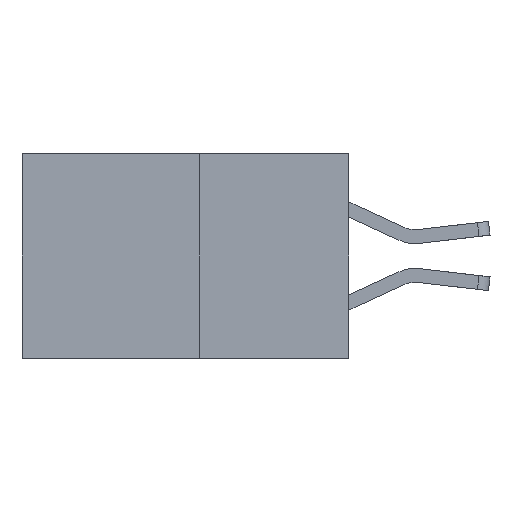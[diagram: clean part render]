
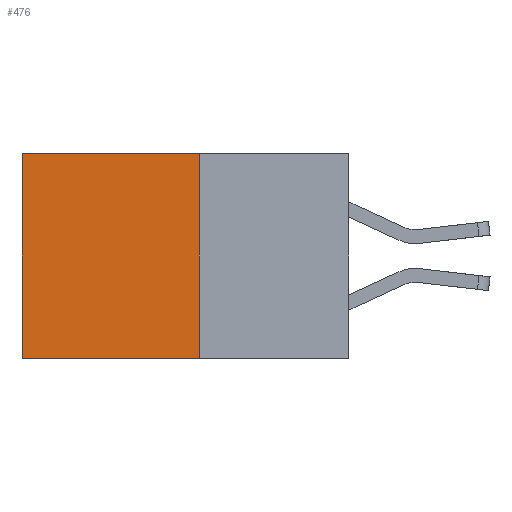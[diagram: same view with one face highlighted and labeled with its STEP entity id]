
A CAD part, left-side view. The second image highlights one B-rep face of the part: STEP entity #476.
In plain terms, the highlighted planar face has unit normal (-1, 0, 0).
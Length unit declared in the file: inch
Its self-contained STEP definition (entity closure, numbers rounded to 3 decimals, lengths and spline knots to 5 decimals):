
#105 = VERTEX_POINT ( 'NONE', #1297 ) ;
#317 = LINE ( 'NONE', #5984, #1931 ) ;
#476 = ADVANCED_FACE ( 'NONE', ( #6765 ), #1693, .F. ) ;
#794 = ORIENTED_EDGE ( 'NONE', *, *, #4523, .T. ) ;
#843 = ORIENTED_EDGE ( 'NONE', *, *, #1957, .F. ) ;
#1030 = DIRECTION ( 'NONE',  ( 0., 0., -1. ) ) ;
#1036 = DIRECTION ( 'NONE',  ( 0., 1., 0. ) ) ;
#1147 = ORIENTED_EDGE ( 'NONE', *, *, #6575, .F. ) ;
#1293 = DIRECTION ( 'NONE',  ( 0., 0., -1. ) ) ;
#1297 = CARTESIAN_POINT ( 'NONE',  ( 0.277, 0.27, -0.37 ) ) ;
#1533 = CARTESIAN_POINT ( 'NONE',  ( 0.277, 0.27, 0. ) ) ;
#1543 = ORIENTED_EDGE ( 'NONE', *, *, #7223, .T. ) ;
#1693 = PLANE ( 'NONE',  #6329 ) ;
#1805 = CARTESIAN_POINT ( 'NONE',  ( 0.277, 0.27, -0.37 ) ) ;
#1931 = VECTOR ( 'NONE', #6585, 39.37008 ) ;
#1957 = EDGE_CURVE ( 'NONE', #105, #7918, #4616, .T. ) ;
#3198 = VECTOR ( 'NONE', #4562, 39.37008 ) ;
#4405 = VECTOR ( 'NONE', #1036, 39.37008 ) ;
#4523 = EDGE_CURVE ( 'NONE', #5938, #7918, #7222, .T. ) ;
#4562 = DIRECTION ( 'NONE',  ( 0., 0., -1. ) ) ;
#4581 = CARTESIAN_POINT ( 'NONE',  ( 0.277, 0.59, -0.37 ) ) ;
#4616 = LINE ( 'NONE', #8134, #4405 ) ;
#4833 = CARTESIAN_POINT ( 'NONE',  ( 0.277, 0.27, -0.37 ) ) ;
#4920 = CARTESIAN_POINT ( 'NONE',  ( 0.277, 0.59, 0. ) ) ;
#5712 = VECTOR ( 'NONE', #1030, 39.37008 ) ;
#5874 = EDGE_LOOP ( 'NONE', ( #794, #843, #1147, #1543 ) ) ;
#5938 = VERTEX_POINT ( 'NONE', #4920 ) ;
#5984 = CARTESIAN_POINT ( 'NONE',  ( 0.277, 0.27, 0. ) ) ;
#6005 = CARTESIAN_POINT ( 'NONE',  ( 0.277, 0.59, -0.37 ) ) ;
#6329 = AXIS2_PLACEMENT_3D ( 'NONE', #1805, #7372, #1293 ) ;
#6368 = VERTEX_POINT ( 'NONE', #1533 ) ;
#6575 = EDGE_CURVE ( 'NONE', #6368, #105, #7285, .T. ) ;
#6585 = DIRECTION ( 'NONE',  ( 0., 1., 0. ) ) ;
#6765 = FACE_OUTER_BOUND ( 'NONE', #5874, .T. ) ;
#7222 = LINE ( 'NONE', #4581, #3198 ) ;
#7223 = EDGE_CURVE ( 'NONE', #6368, #5938, #317, .T. ) ;
#7285 = LINE ( 'NONE', #4833, #5712 ) ;
#7372 = DIRECTION ( 'NONE',  ( 1., 0., 0. ) ) ;
#7918 = VERTEX_POINT ( 'NONE', #6005 ) ;
#8134 = CARTESIAN_POINT ( 'NONE',  ( 0.277, 0.27, -0.37 ) ) ;
